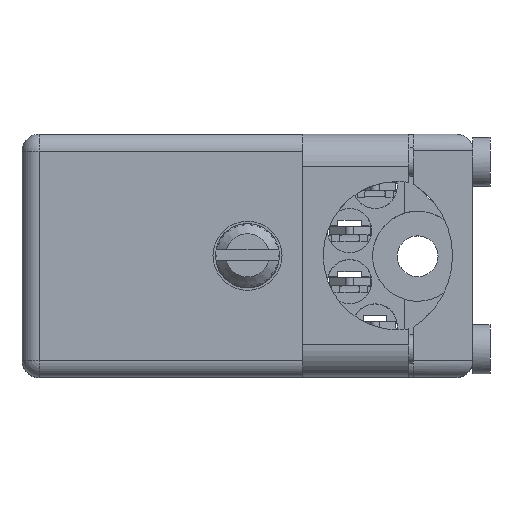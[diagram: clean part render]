
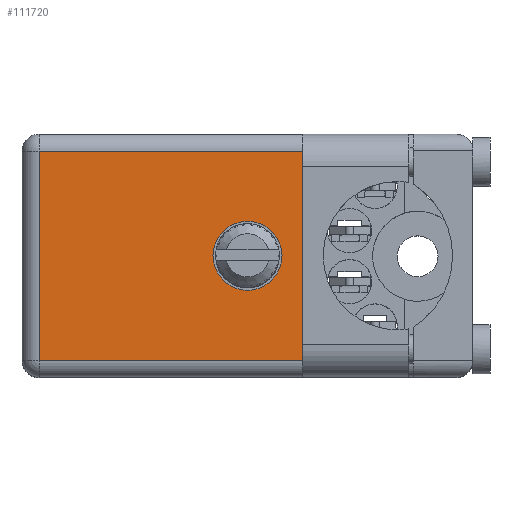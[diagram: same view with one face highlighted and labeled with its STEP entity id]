
A CAD part, top view. The second image highlights one B-rep face of the part: STEP entity #111720.
In plain terms, the highlighted face is planar.
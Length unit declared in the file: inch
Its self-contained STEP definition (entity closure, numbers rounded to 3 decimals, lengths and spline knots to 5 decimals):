
#2186 = ORIENTED_EDGE ( 'NONE', *, *, #110352, .F. ) ;
#3498 = LINE ( 'NONE', #116211, #28783 ) ;
#4024 = AXIS2_PLACEMENT_3D ( 'NONE', #67890, #139076, #37874 ) ;
#14390 = DIRECTION ( 'NONE',  ( -1., 0., 0. ) ) ;
#21456 = CARTESIAN_POINT ( 'NONE',  ( 0.4875, 0.806, -0.3575 ) ) ;
#27907 = EDGE_CURVE ( 'NONE', #103127, #83956, #100243, .T. ) ;
#28783 = VECTOR ( 'NONE', #14390, 39.37008 ) ;
#29152 = VECTOR ( 'NONE', #168498, 39.37008 ) ;
#31485 = CARTESIAN_POINT ( 'NONE',  ( 0., 0.806, 0. ) ) ;
#33559 = CARTESIAN_POINT ( 'NONE',  ( 0.2025, 0.806, -0.245 ) ) ;
#37238 = FACE_BOUND ( 'NONE', #85266, .T. ) ;
#37874 = DIRECTION ( 'NONE',  ( -1., 0., 0. ) ) ;
#39596 = CIRCLE ( 'NONE', #82389, 0.1015 ) ;
#43294 = CARTESIAN_POINT ( 'NONE',  ( -0.6625, 0.806, -0.3075 ) ) ;
#47688 = EDGE_CURVE ( 'NONE', #49663, #91009, #121561, .T. ) ;
#48466 = VERTEX_POINT ( 'NONE', #165566 ) ;
#49663 = VERTEX_POINT ( 'NONE', #130256 ) ;
#49994 = EDGE_CURVE ( 'NONE', #148839, #49663, #128941, .T. ) ;
#51040 = DIRECTION ( 'NONE',  ( 0., 0., 1. ) ) ;
#56765 = DIRECTION ( 'NONE',  ( -1., 0., 0. ) ) ;
#59110 = ORIENTED_EDGE ( 'NONE', *, *, #135073, .F. ) ;
#59821 = CARTESIAN_POINT ( 'NONE',  ( 0.4875, 0.806, 0.3075 ) ) ;
#62583 = CARTESIAN_POINT ( 'NONE',  ( 0.2025, 0.806, 0.245 ) ) ;
#66310 = ORIENTED_EDGE ( 'NONE', *, *, #88138, .T. ) ;
#67890 = CARTESIAN_POINT ( 'NONE',  ( -0.6625, 0.806, -0.3575 ) ) ;
#70121 = ORIENTED_EDGE ( 'NONE', *, *, #49994, .T. ) ;
#73273 = CARTESIAN_POINT ( 'NONE',  ( 0., 0.806, -0.1015 ) ) ;
#74942 = CARTESIAN_POINT ( 'NONE',  ( 0.4875, 0.806, 0.245 ) ) ;
#75845 = ORIENTED_EDGE ( 'NONE', *, *, #155860, .T. ) ;
#75859 = ORIENTED_EDGE ( 'NONE', *, *, #27907, .T. ) ;
#77974 = ORIENTED_EDGE ( 'NONE', *, *, #47688, .T. ) ;
#78506 = CIRCLE ( 'NONE', #184737, 0.1015 ) ;
#79610 = DIRECTION ( 'NONE',  ( 0., 0., 1. ) ) ;
#82389 = AXIS2_PLACEMENT_3D ( 'NONE', #31485, #176253, #103171 ) ;
#82554 = VECTOR ( 'NONE', #85273, 39.37008 ) ;
#83956 = VERTEX_POINT ( 'NONE', #33559 ) ;
#85266 = EDGE_LOOP ( 'NONE', ( #2186, #59110 ) ) ;
#85273 = DIRECTION ( 'NONE',  ( 1., 0., 0. ) ) ;
#87962 = CARTESIAN_POINT ( 'NONE',  ( -0.6125, 0.806, -0.3075 ) ) ;
#88138 = EDGE_CURVE ( 'NONE', #130137, #103127, #3498, .T. ) ;
#89175 = LINE ( 'NONE', #21456, #105378 ) ;
#90897 = CARTESIAN_POINT ( 'NONE',  ( 0.4875, 0.806, -0.245 ) ) ;
#91009 = VERTEX_POINT ( 'NONE', #59821 ) ;
#95379 = CARTESIAN_POINT ( 'NONE',  ( -0.6125, 0.806, -0.3575 ) ) ;
#100243 = LINE ( 'NONE', #123630, #29152 ) ;
#102008 = VERTEX_POINT ( 'NONE', #73273 ) ;
#103127 = VERTEX_POINT ( 'NONE', #62583 ) ;
#103171 = DIRECTION ( 'NONE',  ( 0., 0., 1. ) ) ;
#105378 = VECTOR ( 'NONE', #79610, 39.37008 ) ;
#105543 = EDGE_CURVE ( 'NONE', #48466, #153274, #89175, .T. ) ;
#109555 = CARTESIAN_POINT ( 'NONE',  ( 0.4875, 0.806, 0.3075 ) ) ;
#110352 = EDGE_CURVE ( 'NONE', #183163, #102008, #39596, .T. ) ;
#111720 = ADVANCED_FACE ( 'NONE', ( #131161, #37238 ), #126292, .T. ) ;
#114895 = DIRECTION ( 'NONE',  ( 0., 1., 0. ) ) ;
#115963 = CARTESIAN_POINT ( 'NONE',  ( 0.2025, 0.806, -0.245 ) ) ;
#116211 = CARTESIAN_POINT ( 'NONE',  ( 0.2025, 0.806, 0.245 ) ) ;
#116398 = ORIENTED_EDGE ( 'NONE', *, *, #105543, .F. ) ;
#121561 = LINE ( 'NONE', #109555, #188199 ) ;
#122145 = CARTESIAN_POINT ( 'NONE',  ( 0., 0.806, 0.1015 ) ) ;
#123630 = CARTESIAN_POINT ( 'NONE',  ( 0.2025, 0.806, 0.245 ) ) ;
#123976 = LINE ( 'NONE', #115963, #82554 ) ;
#124981 = DIRECTION ( 'NONE',  ( 1., 0., 0. ) ) ;
#125532 = DIRECTION ( 'NONE',  ( 0., 0., 1. ) ) ;
#126292 = PLANE ( 'NONE',  #4024 ) ;
#128941 = LINE ( 'NONE', #95379, #142637 ) ;
#130137 = VERTEX_POINT ( 'NONE', #74942 ) ;
#130256 = CARTESIAN_POINT ( 'NONE',  ( -0.6125, 0.806, 0.3075 ) ) ;
#130297 = CARTESIAN_POINT ( 'NONE',  ( 0., 0.806, 0. ) ) ;
#131161 = FACE_OUTER_BOUND ( 'NONE', #151975, .T. ) ;
#135073 = EDGE_CURVE ( 'NONE', #102008, #183163, #78506, .T. ) ;
#139076 = DIRECTION ( 'NONE',  ( 0., 1., 0. ) ) ;
#140234 = VECTOR ( 'NONE', #56765, 39.37008 ) ;
#141511 = ORIENTED_EDGE ( 'NONE', *, *, #182865, .F. ) ;
#142521 = ORIENTED_EDGE ( 'NONE', *, *, #168495, .T. ) ;
#142637 = VECTOR ( 'NONE', #125532, 39.37008 ) ;
#145001 = DIRECTION ( 'NONE',  ( 0., 0., 1. ) ) ;
#148839 = VERTEX_POINT ( 'NONE', #87962 ) ;
#151975 = EDGE_LOOP ( 'NONE', ( #70121, #77974, #141511, #66310, #75859, #142521, #116398, #75845 ) ) ;
#153274 = VERTEX_POINT ( 'NONE', #90897 ) ;
#155860 = EDGE_CURVE ( 'NONE', #48466, #148839, #158447, .T. ) ;
#158447 = LINE ( 'NONE', #43294, #140234 ) ;
#165566 = CARTESIAN_POINT ( 'NONE',  ( 0.4875, 0.806, -0.3075 ) ) ;
#167169 = LINE ( 'NONE', #175417, #180952 ) ;
#168495 = EDGE_CURVE ( 'NONE', #83956, #153274, #123976, .T. ) ;
#168498 = DIRECTION ( 'NONE',  ( 0., 0., -1. ) ) ;
#175417 = CARTESIAN_POINT ( 'NONE',  ( 0.4875, 0.806, -0.3575 ) ) ;
#176253 = DIRECTION ( 'NONE',  ( 0., 1., 0. ) ) ;
#180952 = VECTOR ( 'NONE', #51040, 39.37008 ) ;
#182865 = EDGE_CURVE ( 'NONE', #130137, #91009, #167169, .T. ) ;
#183163 = VERTEX_POINT ( 'NONE', #122145 ) ;
#184737 = AXIS2_PLACEMENT_3D ( 'NONE', #130297, #114895, #145001 ) ;
#188199 = VECTOR ( 'NONE', #124981, 39.37008 ) ;
